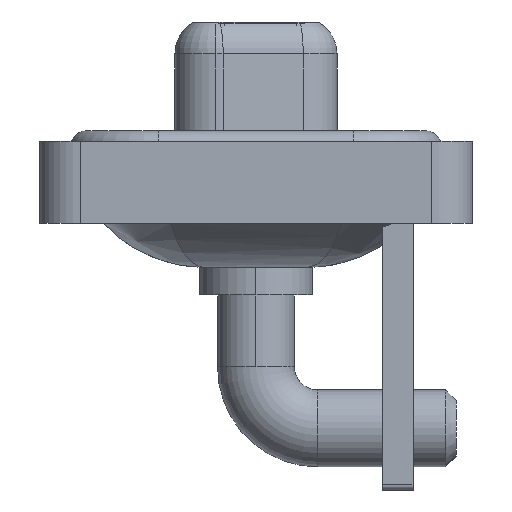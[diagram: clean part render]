
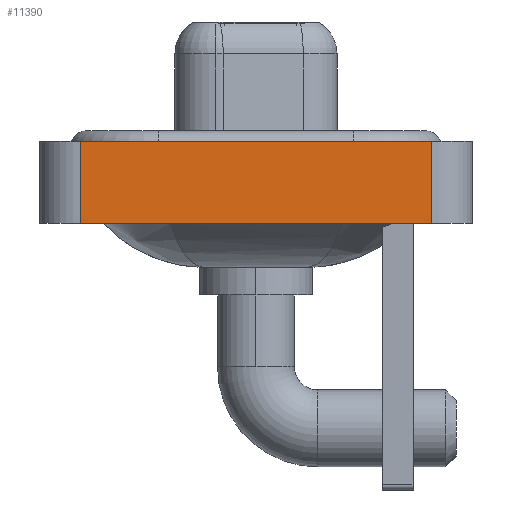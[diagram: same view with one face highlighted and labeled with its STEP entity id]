
A CAD part, left-side view. The second image highlights one B-rep face of the part: STEP entity #11390.
In plain terms, the highlighted planar face has unit normal (-1, 0, 0).
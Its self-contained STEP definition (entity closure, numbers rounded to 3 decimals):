
#186 = VERTEX_POINT ( 'NONE', #12849 ) ;
#258 = VECTOR ( 'NONE', #11011, 1000. ) ;
#671 = LINE ( 'NONE', #16415, #258 ) ;
#679 = DIRECTION ( 'NONE',  ( 0., 0., 1. ) ) ;
#1926 = EDGE_CURVE ( 'NONE', #9462, #6765, #671, .T. ) ;
#2260 = LINE ( 'NONE', #13026, #13824 ) ;
#2437 = DIRECTION ( 'NONE',  ( 0., 0., 1. ) ) ;
#2772 = ORIENTED_EDGE ( 'NONE', *, *, #7656, .T. ) ;
#3074 = LINE ( 'NONE', #16109, #5801 ) ;
#3264 = PLANE ( 'NONE',  #4619 ) ;
#4520 = CARTESIAN_POINT ( 'NONE',  ( -7.3, -8.55, -3.6 ) ) ;
#4619 = AXIS2_PLACEMENT_3D ( 'NONE', #4761, #8309, #7267 ) ;
#4761 = CARTESIAN_POINT ( 'NONE',  ( -7.3, -8.55, -3.6 ) ) ;
#4962 = ORIENTED_EDGE ( 'NONE', *, *, #1926, .F. ) ;
#5801 = VECTOR ( 'NONE', #11022, 1000. ) ;
#6765 = VERTEX_POINT ( 'NONE', #13308 ) ;
#7267 = DIRECTION ( 'NONE',  ( 0., 0., 1. ) ) ;
#7341 = ORIENTED_EDGE ( 'NONE', *, *, #10597, .F. ) ;
#7505 = EDGE_LOOP ( 'NONE', ( #15395, #4962, #7341, #2772 ) ) ;
#7656 = EDGE_CURVE ( 'NONE', #186, #8363, #3074, .T. ) ;
#8309 = DIRECTION ( 'NONE',  ( -1., 0., 0. ) ) ;
#8363 = VERTEX_POINT ( 'NONE', #4520 ) ;
#8366 = CARTESIAN_POINT ( 'NONE',  ( -7.3, 8.55, -3.6 ) ) ;
#9462 = VERTEX_POINT ( 'NONE', #14163 ) ;
#9685 = FACE_OUTER_BOUND ( 'NONE', #7505, .T. ) ;
#9875 = EDGE_CURVE ( 'NONE', #8363, #6765, #2260, .T. ) ;
#10597 = EDGE_CURVE ( 'NONE', #186, #9462, #16423, .T. ) ;
#11011 = DIRECTION ( 'NONE',  ( 0., -1., 0. ) ) ;
#11022 = DIRECTION ( 'NONE',  ( 0., -1., 0. ) ) ;
#11390 = ADVANCED_FACE ( 'NONE', ( #9685 ), #3264, .T. ) ;
#12849 = CARTESIAN_POINT ( 'NONE',  ( -7.3, 8.55, -3.6 ) ) ;
#13026 = CARTESIAN_POINT ( 'NONE',  ( -7.3, -8.55, -3.6 ) ) ;
#13308 = CARTESIAN_POINT ( 'NONE',  ( -7.3, -8.55, 0.4 ) ) ;
#13393 = VECTOR ( 'NONE', #679, 1000. ) ;
#13824 = VECTOR ( 'NONE', #2437, 1000. ) ;
#14163 = CARTESIAN_POINT ( 'NONE',  ( -7.3, 8.55, 0.4 ) ) ;
#15395 = ORIENTED_EDGE ( 'NONE', *, *, #9875, .T. ) ;
#16109 = CARTESIAN_POINT ( 'NONE',  ( -7.3, -8.55, -3.6 ) ) ;
#16415 = CARTESIAN_POINT ( 'NONE',  ( -7.3, -8.55, 0.4 ) ) ;
#16423 = LINE ( 'NONE', #8366, #13393 ) ;
